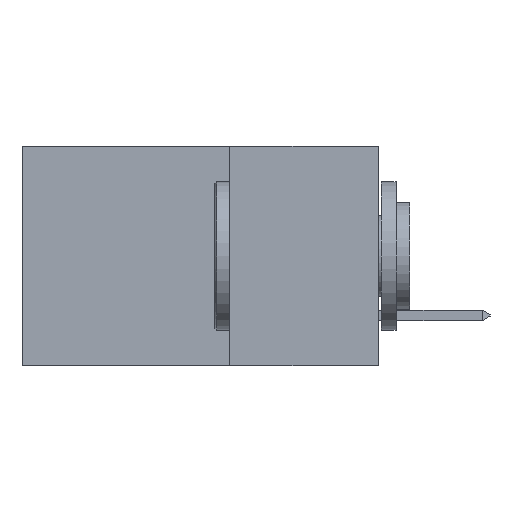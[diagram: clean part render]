
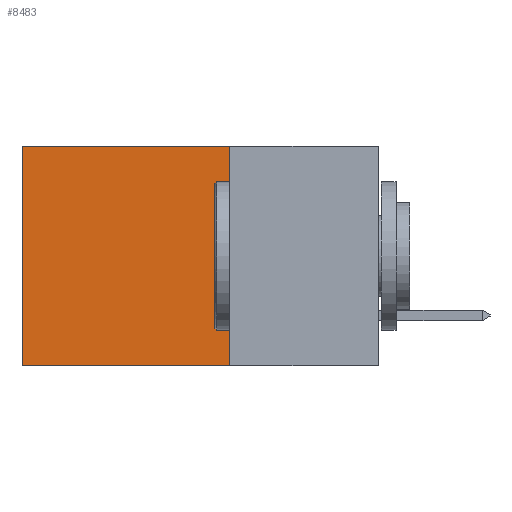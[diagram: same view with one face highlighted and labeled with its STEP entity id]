
A CAD part, left-side view. The second image highlights one B-rep face of the part: STEP entity #8483.
In plain terms, the highlighted planar face has unit normal (-1, 0, 0).
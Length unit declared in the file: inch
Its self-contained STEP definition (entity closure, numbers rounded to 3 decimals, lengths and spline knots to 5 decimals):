
#248 = VERTEX_POINT ( 'NONE', #1348 ) ;
#693 = DIRECTION ( 'NONE',  ( 0., 1., 0. ) ) ;
#896 = LINE ( 'NONE', #7226, #13203 ) ;
#1348 = CARTESIAN_POINT ( 'NONE',  ( 0.298, 0.25, -0.37 ) ) ;
#1715 = LINE ( 'NONE', #15208, #4780 ) ;
#1750 = AXIS2_PLACEMENT_3D ( 'NONE', #13484, #5114, #13542 ) ;
#2001 = VERTEX_POINT ( 'NONE', #9352 ) ;
#3947 = PLANE ( 'NONE',  #1750 ) ;
#4183 = CARTESIAN_POINT ( 'NONE',  ( 0.298, 0.25, 0. ) ) ;
#4424 = EDGE_CURVE ( 'NONE', #248, #14928, #7880, .T. ) ;
#4653 = ORIENTED_EDGE ( 'NONE', *, *, #10482, .F. ) ;
#4780 = VECTOR ( 'NONE', #9259, 39.37008 ) ;
#4954 = CARTESIAN_POINT ( 'NONE',  ( 0.298, 0.6, 0. ) ) ;
#5033 = VECTOR ( 'NONE', #9561, 39.37008 ) ;
#5114 = DIRECTION ( 'NONE',  ( 1., 0., 0. ) ) ;
#5753 = FACE_OUTER_BOUND ( 'NONE', #12799, .T. ) ;
#7226 = CARTESIAN_POINT ( 'NONE',  ( 0.298, 0.6, 0. ) ) ;
#7880 = LINE ( 'NONE', #13038, #5033 ) ;
#8483 = ADVANCED_FACE ( 'NONE', ( #5753 ), #3947, .F. ) ;
#8484 = ORIENTED_EDGE ( 'NONE', *, *, #15047, .T. ) ;
#9259 = DIRECTION ( 'NONE',  ( 0., 0., -1. ) ) ;
#9333 = EDGE_CURVE ( 'NONE', #2001, #13060, #10347, .T. ) ;
#9352 = CARTESIAN_POINT ( 'NONE',  ( 0.298, 0.25, 0. ) ) ;
#9561 = DIRECTION ( 'NONE',  ( 0., 1., 0. ) ) ;
#10347 = LINE ( 'NONE', #4183, #13856 ) ;
#10482 = EDGE_CURVE ( 'NONE', #2001, #248, #1715, .T. ) ;
#10694 = CARTESIAN_POINT ( 'NONE',  ( 0.298, 0.6, -0.37 ) ) ;
#12799 = EDGE_LOOP ( 'NONE', ( #8484, #13720, #4653, #14491 ) ) ;
#13038 = CARTESIAN_POINT ( 'NONE',  ( 0.298, 0.25, -0.37 ) ) ;
#13060 = VERTEX_POINT ( 'NONE', #4954 ) ;
#13203 = VECTOR ( 'NONE', #13279, 39.37008 ) ;
#13279 = DIRECTION ( 'NONE',  ( 0., 0., -1. ) ) ;
#13484 = CARTESIAN_POINT ( 'NONE',  ( 0.298, 0.25, 0. ) ) ;
#13542 = DIRECTION ( 'NONE',  ( 0., 0., -1. ) ) ;
#13720 = ORIENTED_EDGE ( 'NONE', *, *, #4424, .F. ) ;
#13856 = VECTOR ( 'NONE', #693, 39.37008 ) ;
#14491 = ORIENTED_EDGE ( 'NONE', *, *, #9333, .T. ) ;
#14928 = VERTEX_POINT ( 'NONE', #10694 ) ;
#15047 = EDGE_CURVE ( 'NONE', #13060, #14928, #896, .T. ) ;
#15208 = CARTESIAN_POINT ( 'NONE',  ( 0.298, 0.25, 0. ) ) ;
